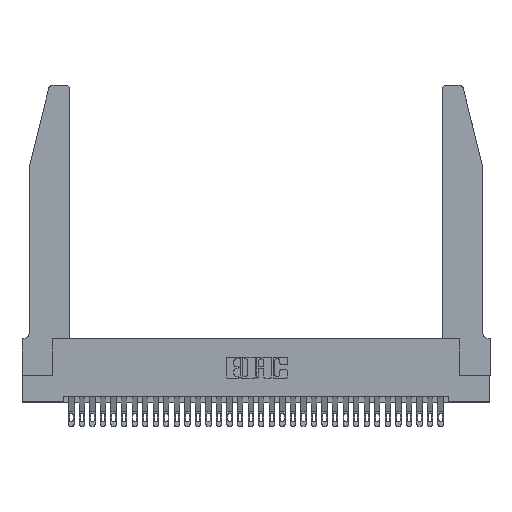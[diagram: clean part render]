
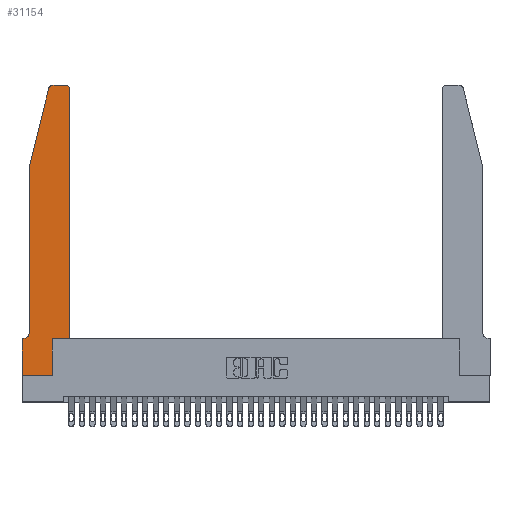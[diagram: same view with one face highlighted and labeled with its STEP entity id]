
A CAD part, top view. The second image highlights one B-rep face of the part: STEP entity #31154.
In plain terms, the highlighted planar face has unit normal (0, 0, 1).
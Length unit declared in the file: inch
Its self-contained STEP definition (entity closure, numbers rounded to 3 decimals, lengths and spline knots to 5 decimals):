
#594 = LINE ( 'NONE', #9807, #9734 ) ;
#998 = VERTEX_POINT ( 'NONE', #6825 ) ;
#1591 = VECTOR ( 'NONE', #30006, 39.37008 ) ;
#1954 = EDGE_CURVE ( 'NONE', #32654, #998, #2387, .T. ) ;
#1998 = ORIENTED_EDGE ( 'NONE', *, *, #33551, .T. ) ;
#2302 = DIRECTION ( 'NONE',  ( -1., 0., 0. ) ) ;
#2335 = ORIENTED_EDGE ( 'NONE', *, *, #8451, .T. ) ;
#2387 = LINE ( 'NONE', #19535, #20913 ) ;
#2514 = DIRECTION ( 'NONE',  ( 0., 0., 1. ) ) ;
#2719 = DIRECTION ( 'NONE',  ( 0., 0., 1. ) ) ;
#2736 = AXIS2_PLACEMENT_3D ( 'NONE', #28619, #2514, #18383 ) ;
#2974 = CIRCLE ( 'NONE', #16662, 0.07 ) ;
#3173 = EDGE_CURVE ( 'NONE', #9687, #8349, #594, .T. ) ;
#3311 = ORIENTED_EDGE ( 'NONE', *, *, #9612, .T. ) ;
#3742 = CARTESIAN_POINT ( 'NONE',  ( 0.0755, 2., 0.37 ) ) ;
#4287 = LINE ( 'NONE', #8605, #19969 ) ;
#4505 = CARTESIAN_POINT ( 'NONE',  ( 0.4205, 2.75, 0.37 ) ) ;
#5171 = CARTESIAN_POINT ( 'NONE',  ( 0.0755, 0.35, 0.37 ) ) ;
#6825 = CARTESIAN_POINT ( 'NONE',  ( 0.4505, 0.35, 0.37 ) ) ;
#6966 = ORIENTED_EDGE ( 'NONE', *, *, #15598, .T. ) ;
#7309 = LINE ( 'NONE', #29316, #18425 ) ;
#7418 = EDGE_LOOP ( 'NONE', ( #13600, #14177, #25067, #9606, #6966, #2335, #3311, #1998, #30712, #31556, #8328, #33438 ) ) ;
#8328 = ORIENTED_EDGE ( 'NONE', *, *, #14240, .T. ) ;
#8349 = VERTEX_POINT ( 'NONE', #25047 ) ;
#8451 = EDGE_CURVE ( 'NONE', #11249, #26672, #23832, .T. ) ;
#8605 = CARTESIAN_POINT ( 'NONE',  ( 0.4505, 0.35, 0.37 ) ) ;
#8906 = AXIS2_PLACEMENT_3D ( 'NONE', #21352, #2719, #23786 ) ;
#8958 = DIRECTION ( 'NONE',  ( 1., 0., 0. ) ) ;
#9487 = VERTEX_POINT ( 'NONE', #18873 ) ;
#9606 = ORIENTED_EDGE ( 'NONE', *, *, #18503, .T. ) ;
#9612 = EDGE_CURVE ( 'NONE', #26672, #11630, #7309, .T. ) ;
#9687 = VERTEX_POINT ( 'NONE', #4505 ) ;
#9734 = VECTOR ( 'NONE', #12523, 39.37008 ) ;
#9807 = CARTESIAN_POINT ( 'NONE',  ( 0.2605, 2.75, 0.37 ) ) ;
#10413 = CARTESIAN_POINT ( 'NONE',  ( 0.0055, 0.35, 0.37 ) ) ;
#11249 = VERTEX_POINT ( 'NONE', #10413 ) ;
#11630 = VERTEX_POINT ( 'NONE', #16218 ) ;
#12104 = DIRECTION ( 'NONE',  ( 0., 0., -1. ) ) ;
#12523 = DIRECTION ( 'NONE',  ( -1., 0., 0. ) ) ;
#12583 = CARTESIAN_POINT ( 'NONE',  ( 0.25487, 2.72718, 0.37 ) ) ;
#12936 = EDGE_CURVE ( 'NONE', #8349, #13369, #16704, .T. ) ;
#13369 = VERTEX_POINT ( 'NONE', #12583 ) ;
#13600 = ORIENTED_EDGE ( 'NONE', *, *, #3173, .T. ) ;
#13715 = AXIS2_PLACEMENT_3D ( 'NONE', #16005, #21622, #29424 ) ;
#13778 = DIRECTION ( 'NONE',  ( 0., 1., 0. ) ) ;
#14177 = ORIENTED_EDGE ( 'NONE', *, *, #12936, .T. ) ;
#14195 = DIRECTION ( 'NONE',  ( 0., -1., 0. ) ) ;
#14240 = EDGE_CURVE ( 'NONE', #998, #18055, #4287, .T. ) ;
#14791 = LINE ( 'NONE', #32903, #1591 ) ;
#15164 = VECTOR ( 'NONE', #2302, 39.37008 ) ;
#15598 = EDGE_CURVE ( 'NONE', #25704, #11249, #2974, .T. ) ;
#15743 = CARTESIAN_POINT ( 'NONE',  ( 0., 0.35, 0.37 ) ) ;
#16005 = CARTESIAN_POINT ( 'NONE',  ( 0.4205, 2.72, 0.37 ) ) ;
#16218 = CARTESIAN_POINT ( 'NONE',  ( 0., 0., 0.37 ) ) ;
#16662 = AXIS2_PLACEMENT_3D ( 'NONE', #33183, #12104, #20052 ) ;
#16704 = CIRCLE ( 'NONE', #8906, 0.03 ) ;
#17976 = EDGE_CURVE ( 'NONE', #13369, #22512, #33853, .T. ) ;
#18055 = VERTEX_POINT ( 'NONE', #30678 ) ;
#18383 = DIRECTION ( 'NONE',  ( 1., 0., 0. ) ) ;
#18425 = VECTOR ( 'NONE', #24085, 39.37008 ) ;
#18503 = EDGE_CURVE ( 'NONE', #22512, #25704, #28821, .T. ) ;
#18747 = CIRCLE ( 'NONE', #13715, 0.03 ) ;
#18873 = CARTESIAN_POINT ( 'NONE',  ( 0.2865, 0., 0.37 ) ) ;
#18978 = VECTOR ( 'NONE', #27128, 39.37008 ) ;
#19535 = CARTESIAN_POINT ( 'NONE',  ( 0.4505, 0.35, 0.37 ) ) ;
#19905 = EDGE_CURVE ( 'NONE', #9487, #32654, #14791, .T. ) ;
#19969 = VECTOR ( 'NONE', #13778, 39.37008 ) ;
#20052 = DIRECTION ( 'NONE',  ( -1., 0., 0. ) ) ;
#20066 = CARTESIAN_POINT ( 'NONE',  ( 0.0755, 2., 0.37 ) ) ;
#20824 = PLANE ( 'NONE',  #2736 ) ;
#20913 = VECTOR ( 'NONE', #8958, 39.37008 ) ;
#21352 = CARTESIAN_POINT ( 'NONE',  ( 0.284, 2.72, 0.37 ) ) ;
#21542 = CARTESIAN_POINT ( 'NONE',  ( 0., 0., 0.37 ) ) ;
#21622 = DIRECTION ( 'NONE',  ( 0., 0., 1. ) ) ;
#21848 = CARTESIAN_POINT ( 'NONE',  ( 0.0755, 2., 0.37 ) ) ;
#21949 = VECTOR ( 'NONE', #26810, 39.37008 ) ;
#22385 = LINE ( 'NONE', #21542, #21949 ) ;
#22512 = VERTEX_POINT ( 'NONE', #20066 ) ;
#23786 = DIRECTION ( 'NONE',  ( 1., 0., 0. ) ) ;
#23832 = LINE ( 'NONE', #5171, #15164 ) ;
#24085 = DIRECTION ( 'NONE',  ( 0., -1., 0. ) ) ;
#25047 = CARTESIAN_POINT ( 'NONE',  ( 0.284, 2.75, 0.37 ) ) ;
#25067 = ORIENTED_EDGE ( 'NONE', *, *, #17976, .T. ) ;
#25704 = VERTEX_POINT ( 'NONE', #29153 ) ;
#26672 = VERTEX_POINT ( 'NONE', #15743 ) ;
#26810 = DIRECTION ( 'NONE',  ( 1., 0., 0. ) ) ;
#27128 = DIRECTION ( 'NONE',  ( -0.239, -0.971, 0. ) ) ;
#28407 = VECTOR ( 'NONE', #14195, 39.37008 ) ;
#28619 = CARTESIAN_POINT ( 'NONE',  ( 0., 0.35, 0.37 ) ) ;
#28694 = EDGE_CURVE ( 'NONE', #18055, #9687, #18747, .T. ) ;
#28821 = LINE ( 'NONE', #3742, #28407 ) ;
#29153 = CARTESIAN_POINT ( 'NONE',  ( 0.0755, 0.42, 0.37 ) ) ;
#29316 = CARTESIAN_POINT ( 'NONE',  ( 0., 0., 0.37 ) ) ;
#29424 = DIRECTION ( 'NONE',  ( 1., 0., 0. ) ) ;
#30006 = DIRECTION ( 'NONE',  ( 0., 1., 0. ) ) ;
#30379 = FACE_OUTER_BOUND ( 'NONE', #7418, .T. ) ;
#30678 = CARTESIAN_POINT ( 'NONE',  ( 0.4505, 2.72, 0.37 ) ) ;
#30712 = ORIENTED_EDGE ( 'NONE', *, *, #19905, .T. ) ;
#30832 = CARTESIAN_POINT ( 'NONE',  ( 0.2865, 0.35, 0.37 ) ) ;
#31154 = ADVANCED_FACE ( 'NONE', ( #30379 ), #20824, .T. ) ;
#31556 = ORIENTED_EDGE ( 'NONE', *, *, #1954, .T. ) ;
#32654 = VERTEX_POINT ( 'NONE', #30832 ) ;
#32903 = CARTESIAN_POINT ( 'NONE',  ( 0.2865, 0.35, 0.37 ) ) ;
#33183 = CARTESIAN_POINT ( 'NONE',  ( 0.0055, 0.42, 0.37 ) ) ;
#33438 = ORIENTED_EDGE ( 'NONE', *, *, #28694, .T. ) ;
#33551 = EDGE_CURVE ( 'NONE', #11630, #9487, #22385, .T. ) ;
#33853 = LINE ( 'NONE', #21848, #18978 ) ;
